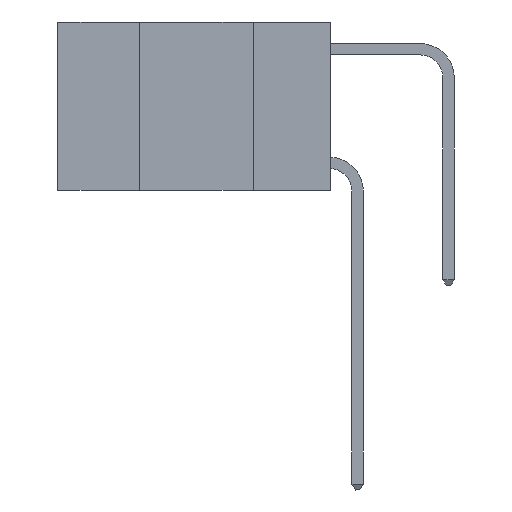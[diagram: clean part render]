
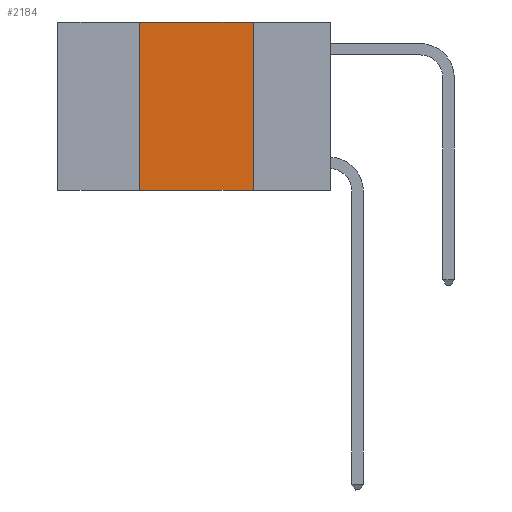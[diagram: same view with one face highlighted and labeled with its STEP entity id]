
A CAD part, left-side view. The second image highlights one B-rep face of the part: STEP entity #2184.
In plain terms, the highlighted planar face has unit normal (-1, 0, 0).
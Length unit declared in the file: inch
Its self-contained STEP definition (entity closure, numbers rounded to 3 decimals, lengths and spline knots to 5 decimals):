
#322 = VECTOR ( 'NONE', #26267, 39.37008 ) ;
#2044 = LINE ( 'NONE', #17348, #14427 ) ;
#2184 = ADVANCED_FACE ( 'NONE', ( #31856 ), #15646, .F. ) ;
#2636 = DIRECTION ( 'NONE',  ( 0., 0., 1. ) ) ;
#3310 = DIRECTION ( 'NONE',  ( 0., 0., -1. ) ) ;
#4921 = EDGE_CURVE ( 'NONE', #8449, #24931, #13619, .T. ) ;
#5034 = DIRECTION ( 'NONE',  ( 0., 0., -1. ) ) ;
#5562 = ORIENTED_EDGE ( 'NONE', *, *, #4921, .F. ) ;
#5587 = CARTESIAN_POINT ( 'NONE',  ( 0., 0.17, 0. ) ) ;
#6389 = LINE ( 'NONE', #15632, #19523 ) ;
#7113 = ORIENTED_EDGE ( 'NONE', *, *, #22282, .F. ) ;
#7247 = AXIS2_PLACEMENT_3D ( 'NONE', #30367, #18103, #3310 ) ;
#7952 = EDGE_LOOP ( 'NONE', ( #7113, #9293, #5562, #11513 ) ) ;
#8449 = VERTEX_POINT ( 'NONE', #27797 ) ;
#9039 = CARTESIAN_POINT ( 'NONE',  ( 0., 0.6, 0. ) ) ;
#9293 = ORIENTED_EDGE ( 'NONE', *, *, #18443, .F. ) ;
#10646 = DIRECTION ( 'NONE',  ( 0., -1., 0. ) ) ;
#11513 = ORIENTED_EDGE ( 'NONE', *, *, #30746, .T. ) ;
#12469 = CARTESIAN_POINT ( 'NONE',  ( 0., 0.42, 0. ) ) ;
#13619 = LINE ( 'NONE', #12469, #25908 ) ;
#14427 = VECTOR ( 'NONE', #5034, 39.37008 ) ;
#15632 = CARTESIAN_POINT ( 'NONE',  ( 0., 0.6, -0.37 ) ) ;
#15646 = PLANE ( 'NONE',  #7247 ) ;
#17348 = CARTESIAN_POINT ( 'NONE',  ( 0., 0.17, 0. ) ) ;
#18103 = DIRECTION ( 'NONE',  ( 1., 0., 0. ) ) ;
#18443 = EDGE_CURVE ( 'NONE', #24931, #21807, #26593, .T. ) ;
#19517 = CARTESIAN_POINT ( 'NONE',  ( 0., 0.42, 0. ) ) ;
#19523 = VECTOR ( 'NONE', #10646, 39.37008 ) ;
#21807 = VERTEX_POINT ( 'NONE', #5587 ) ;
#22282 = EDGE_CURVE ( 'NONE', #21807, #24294, #2044, .T. ) ;
#24294 = VERTEX_POINT ( 'NONE', #31911 ) ;
#24931 = VERTEX_POINT ( 'NONE', #19517 ) ;
#25908 = VECTOR ( 'NONE', #2636, 39.37008 ) ;
#26267 = DIRECTION ( 'NONE',  ( 0., -1., 0. ) ) ;
#26593 = LINE ( 'NONE', #9039, #322 ) ;
#27797 = CARTESIAN_POINT ( 'NONE',  ( 0., 0.42, -0.37 ) ) ;
#30367 = CARTESIAN_POINT ( 'NONE',  ( 0., 0.6, 0. ) ) ;
#30746 = EDGE_CURVE ( 'NONE', #8449, #24294, #6389, .T. ) ;
#31856 = FACE_OUTER_BOUND ( 'NONE', #7952, .T. ) ;
#31911 = CARTESIAN_POINT ( 'NONE',  ( 0., 0.17, -0.37 ) ) ;
